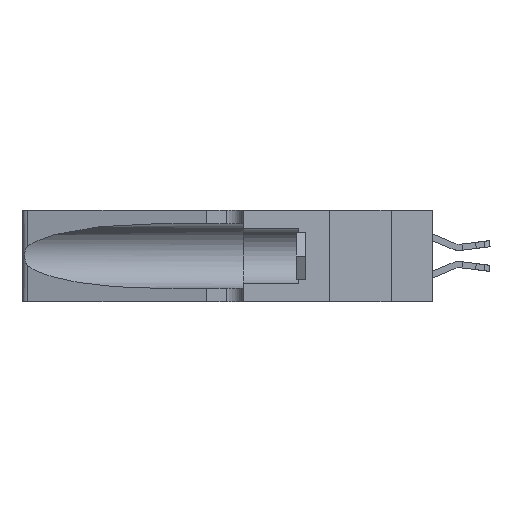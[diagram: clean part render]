
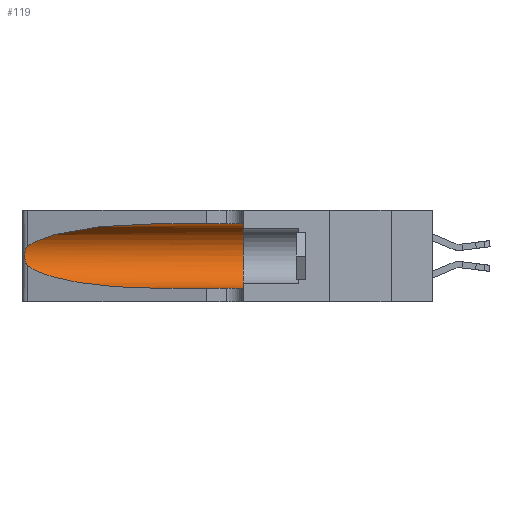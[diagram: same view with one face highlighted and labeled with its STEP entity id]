
A CAD part, left-side view. The second image highlights one B-rep face of the part: STEP entity #119.
In plain terms, the highlighted cylindrical face has radius 3.308 mm (diameter 6.617 mm), a partial arc.
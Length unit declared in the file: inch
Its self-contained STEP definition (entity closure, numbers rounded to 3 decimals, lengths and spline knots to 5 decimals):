
#119 = ADVANCED_FACE ( 'NONE', ( #1884 ), #21869, .F. ) ;
#294 = ORIENTED_EDGE ( 'NONE', *, *, #22952, .T. ) ;
#734 = CARTESIAN_POINT ( 'NONE',  ( 0.25789, 1.23486, 0.15765 ) ) ;
#1884 = FACE_OUTER_BOUND ( 'NONE', #24028, .T. ) ;
#2146 = CARTESIAN_POINT ( 'NONE',  ( 0.2373, 1.15595, 0.28018 ) ) ;
#2359 = DIRECTION ( 'NONE',  ( 0., 0., -1. ) ) ;
#2630 = AXIS2_PLACEMENT_3D ( 'NONE', #25526, #10013, #28130 ) ;
#3379 = CARTESIAN_POINT ( 'NONE',  ( 0.25555, 1.22993, 0.14849 ) ) ;
#3460 = EDGE_CURVE ( 'NONE', #5171, #16824, #17005, .T. ) ;
#3556 = VECTOR ( 'NONE', #25144, 39.37008 ) ;
#4294 = ORIENTED_EDGE ( 'NONE', *, *, #21668, .F. ) ;
#4404 = DIRECTION ( 'NONE',  ( 0., -1., 0. ) ) ;
#5171 = VERTEX_POINT ( 'NONE', #18206 ) ;
#5269 = CARTESIAN_POINT ( 'NONE',  ( 0.1305, 0.72297, 0.31525 ) ) ;
#5374 = VERTEX_POINT ( 'NONE', #21573 ) ;
#5879 = CARTESIAN_POINT ( 'NONE',  ( 0.25555, 1.22994, 0.2215 ) ) ;
#5969 = VERTEX_POINT ( 'NONE', #8343 ) ;
#7295 = AXIS2_PLACEMENT_3D ( 'NONE', #10778, #4404, #2359 ) ;
#8190 = CARTESIAN_POINT ( 'NONE',  ( 0.25487, 1.22718, 0.14631 ) ) ;
#8343 = CARTESIAN_POINT ( 'NONE',  ( 0.1305, 0.72297, 0.05475 ) ) ;
#8517 = CARTESIAN_POINT ( 'NONE',  ( 0.25787, 1.23484, 0.2124 ) ) ;
#9144 = VECTOR ( 'NONE', #26887, 39.37008 ) ;
#10013 = DIRECTION ( 'NONE',  ( 0., 1., 0. ) ) ;
#10778 = CARTESIAN_POINT ( 'NONE',  ( 0.1305, 1.61858, 0.185 ) ) ;
#11133 = CARTESIAN_POINT ( 'NONE',  ( 0.26018, 1.23835, 0.19895 ) ) ;
#11783 =( BOUNDED_CURVE ( )  B_SPLINE_CURVE ( 3, ( #8190, #26328, #28929, #13440 ),
 .UNSPECIFIED., .F., .T. ) 
 B_SPLINE_CURVE_WITH_KNOTS ( ( 4, 4 ),
 ( 3.44316, 4.71239 ),
 .UNSPECIFIED. ) 
 CURVE ( )  GEOMETRIC_REPRESENTATION_ITEM ( )  RATIONAL_B_SPLINE_CURVE ( ( 1., 0.87, 0.87, 1. ) ) 
 REPRESENTATION_ITEM ( '' )  );
#12922 = CIRCLE ( 'NONE', #2630, 0.13025 ) ;
#13440 = CARTESIAN_POINT ( 'NONE',  ( 0.1305, 0.72297, 0.05475 ) ) ;
#13771 = CARTESIAN_POINT ( 'NONE',  ( 0.26075, 1.23896, 0.178 ) ) ;
#14336 = ORIENTED_EDGE ( 'NONE', *, *, #3460, .T. ) ;
#14425 = ORIENTED_EDGE ( 'NONE', *, *, #23181, .T. ) ;
#14778 = ORIENTED_EDGE ( 'NONE', *, *, #23330, .T. ) ;
#14943 = CARTESIAN_POINT ( 'NONE',  ( 0.25487, 1.22718, 0.14631 ) ) ;
#16078 = LINE ( 'NONE', #21731, #9144 ) ;
#16389 = CARTESIAN_POINT ( 'NONE',  ( 0.25856, 1.23593, 0.16098 ) ) ;
#16824 = VERTEX_POINT ( 'NONE', #14943 ) ;
#17005 = B_SPLINE_CURVE_WITH_KNOTS ( 'NONE', 3,
 ( #29149, #5879, #24052, #8517, #26647, #11133, #29252, #13771, #31852, #16389, #734, #19006, #3379, #21592 ),
 .UNSPECIFIED., .F., .F.,
 ( 4, 2, 2, 2, 2, 2, 4 ),
 ( 0., 0.00027, 0.00053, 0.00107, 0.0016, 0.00187, 0.00214 ),
 .UNSPECIFIED. ) ;
#17449 = LINE ( 'NONE', #19987, #3556 ) ;
#18205 = EDGE_CURVE ( 'NONE', #29606, #25432, #17449, .T. ) ;
#18206 = CARTESIAN_POINT ( 'NONE',  ( 0.25487, 1.22718, 0.22369 ) ) ;
#19006 = CARTESIAN_POINT ( 'NONE',  ( 0.25639, 1.23186, 0.15144 ) ) ;
#19987 = CARTESIAN_POINT ( 'NONE',  ( 0.1305, 1.61858, 0.31525 ) ) ;
#20398 = CARTESIAN_POINT ( 'NONE',  ( 0.25487, 1.22718, 0.22369 ) ) ;
#20904 =( BOUNDED_CURVE ( )  B_SPLINE_CURVE ( 3, ( #33238, #28039, #2146, #20398 ),
 .UNSPECIFIED., .F., .T. ) 
 B_SPLINE_CURVE_WITH_KNOTS ( ( 4, 4 ),
 ( 1.5708, 2.84003 ),
 .UNSPECIFIED. ) 
 CURVE ( )  GEOMETRIC_REPRESENTATION_ITEM ( )  RATIONAL_B_SPLINE_CURVE ( ( 1., 0.87, 0.87, 1. ) ) 
 REPRESENTATION_ITEM ( '' )  );
#21542 = ORIENTED_EDGE ( 'NONE', *, *, #18205, .F. ) ;
#21573 = CARTESIAN_POINT ( 'NONE',  ( 0.1305, 0.35, 0.05475 ) ) ;
#21592 = CARTESIAN_POINT ( 'NONE',  ( 0.25487, 1.22718, 0.14631 ) ) ;
#21668 = EDGE_CURVE ( 'NONE', #25432, #5374, #12922, .T. ) ;
#21731 = CARTESIAN_POINT ( 'NONE',  ( 0.1305, 1.61858, 0.05475 ) ) ;
#21869 = CYLINDRICAL_SURFACE ( 'NONE', #7295, 0.13025 ) ;
#22952 = EDGE_CURVE ( 'NONE', #29606, #5171, #20904, .T. ) ;
#23181 = EDGE_CURVE ( 'NONE', #16824, #5969, #11783, .T. ) ;
#23330 = EDGE_CURVE ( 'NONE', #5969, #5374, #16078, .T. ) ;
#24028 = EDGE_LOOP ( 'NONE', ( #294, #14336, #14425, #14778, #4294, #21542 ) ) ;
#24052 = CARTESIAN_POINT ( 'NONE',  ( 0.25639, 1.23184, 0.21858 ) ) ;
#25144 = DIRECTION ( 'NONE',  ( 0., -1., 0. ) ) ;
#25183 = CARTESIAN_POINT ( 'NONE',  ( 0.1305, 0.35, 0.31525 ) ) ;
#25432 = VERTEX_POINT ( 'NONE', #25183 ) ;
#25526 = CARTESIAN_POINT ( 'NONE',  ( 0.1305, 0.35, 0.185 ) ) ;
#26328 = CARTESIAN_POINT ( 'NONE',  ( 0.2373, 1.15595, 0.08982 ) ) ;
#26647 = CARTESIAN_POINT ( 'NONE',  ( 0.25854, 1.2359, 0.20912 ) ) ;
#26887 = DIRECTION ( 'NONE',  ( 0., -1., 0. ) ) ;
#28039 = CARTESIAN_POINT ( 'NONE',  ( 0.18966, 0.96281, 0.31525 ) ) ;
#28130 = DIRECTION ( 'NONE',  ( 0., 0., 1. ) ) ;
#28929 = CARTESIAN_POINT ( 'NONE',  ( 0.18966, 0.96281, 0.05475 ) ) ;
#29149 = CARTESIAN_POINT ( 'NONE',  ( 0.25487, 1.22718, 0.22369 ) ) ;
#29252 = CARTESIAN_POINT ( 'NONE',  ( 0.26075, 1.23896, 0.19203 ) ) ;
#29606 = VERTEX_POINT ( 'NONE', #5269 ) ;
#31852 = CARTESIAN_POINT ( 'NONE',  ( 0.26017, 1.23833, 0.17102 ) ) ;
#33238 = CARTESIAN_POINT ( 'NONE',  ( 0.1305, 0.72297, 0.31525 ) ) ;
